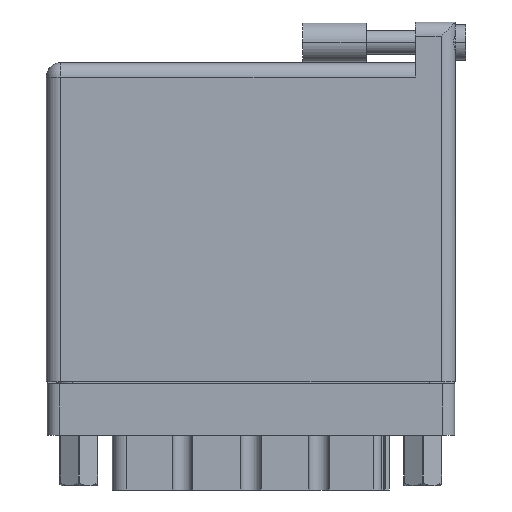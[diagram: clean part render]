
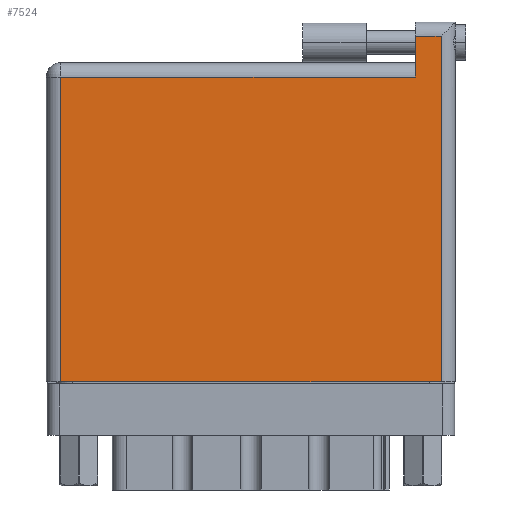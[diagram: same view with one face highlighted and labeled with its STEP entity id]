
A CAD part, front view. The second image highlights one B-rep face of the part: STEP entity #7524.
In plain terms, the highlighted face is planar.
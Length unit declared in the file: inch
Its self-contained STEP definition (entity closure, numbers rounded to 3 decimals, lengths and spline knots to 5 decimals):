
#663 = ORIENTED_EDGE ( 'NONE', *, *, #12104, .T. ) ;
#1580 = CARTESIAN_POINT ( 'NONE',  ( 0.07, 1.496, 0. ) ) ;
#2237 = EDGE_CURVE ( 'NONE', #16947, #13830, #30861, .T. ) ;
#3186 = CARTESIAN_POINT ( 'NONE',  ( 0.07, 0., 0. ) ) ;
#3927 = DIRECTION ( 'NONE',  ( -1., 0., 0. ) ) ;
#3992 = CARTESIAN_POINT ( 'NONE',  ( 1.811, 1.496, 0. ) ) ;
#4603 = VECTOR ( 'NONE', #3927, 39.37008 ) ;
#5456 = EDGE_CURVE ( 'NONE', #15926, #28060, #41928, .T. ) ;
#6960 = LINE ( 'NONE', #19042, #4603 ) ;
#7524 = ADVANCED_FACE ( 'NONE', ( #47416 ), #20236, .F. ) ;
#8423 = DIRECTION ( 'NONE',  ( 0., 0., -1. ) ) ;
#9337 = CARTESIAN_POINT ( 'NONE',  ( 1.811, 1.766, 0. ) ) ;
#10677 = VECTOR ( 'NONE', #40024, 39.37008 ) ;
#11774 = CARTESIAN_POINT ( 'NONE',  ( 0., 1.496, 0. ) ) ;
#11932 = ORIENTED_EDGE ( 'NONE', *, *, #20162, .T. ) ;
#12104 = EDGE_CURVE ( 'NONE', #13830, #31296, #29104, .T. ) ;
#12334 = CARTESIAN_POINT ( 'NONE',  ( 1.811, 1.696, 0. ) ) ;
#13830 = VERTEX_POINT ( 'NONE', #1580 ) ;
#14133 = DIRECTION ( 'NONE',  ( 1., 0., 0. ) ) ;
#14716 = CARTESIAN_POINT ( 'NONE',  ( 1.938, 0., 0. ) ) ;
#15600 = VECTOR ( 'NONE', #42446, 39.37008 ) ;
#15926 = VERTEX_POINT ( 'NONE', #14716 ) ;
#16239 = DIRECTION ( 'NONE',  ( -1., 0., 0. ) ) ;
#16947 = VERTEX_POINT ( 'NONE', #3992 ) ;
#19042 = CARTESIAN_POINT ( 'NONE',  ( 0., 1.696, 0. ) ) ;
#20162 = EDGE_CURVE ( 'NONE', #25315, #16947, #20654, .T. ) ;
#20236 = PLANE ( 'NONE',  #43558 ) ;
#20470 = ORIENTED_EDGE ( 'NONE', *, *, #5456, .T. ) ;
#20654 = LINE ( 'NONE', #9337, #10677 ) ;
#20700 = VECTOR ( 'NONE', #14133, 39.37008 ) ;
#25315 = VERTEX_POINT ( 'NONE', #12334 ) ;
#26406 = ORIENTED_EDGE ( 'NONE', *, *, #2237, .T. ) ;
#27070 = CARTESIAN_POINT ( 'NONE',  ( 1.938, 1.696, 0. ) ) ;
#27902 = EDGE_CURVE ( 'NONE', #28060, #25315, #6960, .T. ) ;
#28060 = VERTEX_POINT ( 'NONE', #27070 ) ;
#28408 = VECTOR ( 'NONE', #38153, 39.37008 ) ;
#29104 = LINE ( 'NONE', #3186, #49383 ) ;
#29453 = CARTESIAN_POINT ( 'NONE',  ( 0.07, 0., 0. ) ) ;
#29945 = EDGE_CURVE ( 'NONE', #31296, #15926, #32471, .T. ) ;
#30861 = LINE ( 'NONE', #11774, #15600 ) ;
#31296 = VERTEX_POINT ( 'NONE', #29453 ) ;
#32471 = LINE ( 'NONE', #48332, #20700 ) ;
#35829 = CARTESIAN_POINT ( 'NONE',  ( 0., 1.566, 0. ) ) ;
#37842 = ORIENTED_EDGE ( 'NONE', *, *, #29945, .T. ) ;
#38153 = DIRECTION ( 'NONE',  ( 0., 1., 0. ) ) ;
#40024 = DIRECTION ( 'NONE',  ( 0., -1., 0. ) ) ;
#41928 = LINE ( 'NONE', #46202, #28408 ) ;
#42446 = DIRECTION ( 'NONE',  ( -1., 0., 0. ) ) ;
#42629 = EDGE_LOOP ( 'NONE', ( #37842, #20470, #43956, #11932, #26406, #663 ) ) ;
#43558 = AXIS2_PLACEMENT_3D ( 'NONE', #35829, #8423, #16239 ) ;
#43956 = ORIENTED_EDGE ( 'NONE', *, *, #27902, .T. ) ;
#44461 = DIRECTION ( 'NONE',  ( 0., -1., 0. ) ) ;
#46202 = CARTESIAN_POINT ( 'NONE',  ( 1.938, 1.766, 0. ) ) ;
#47416 = FACE_OUTER_BOUND ( 'NONE', #42629, .T. ) ;
#48332 = CARTESIAN_POINT ( 'NONE',  ( 0., 0., 0. ) ) ;
#49383 = VECTOR ( 'NONE', #44461, 39.37008 ) ;
